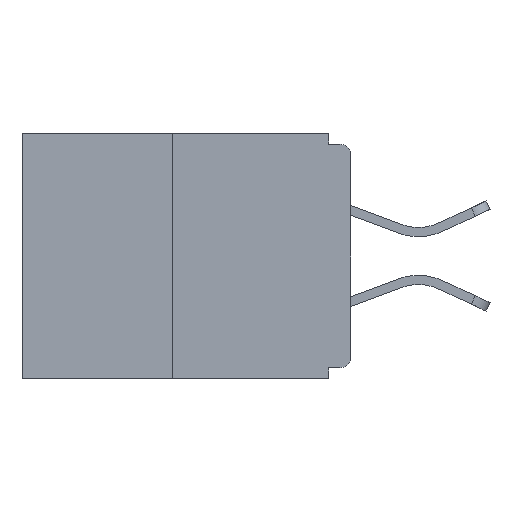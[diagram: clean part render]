
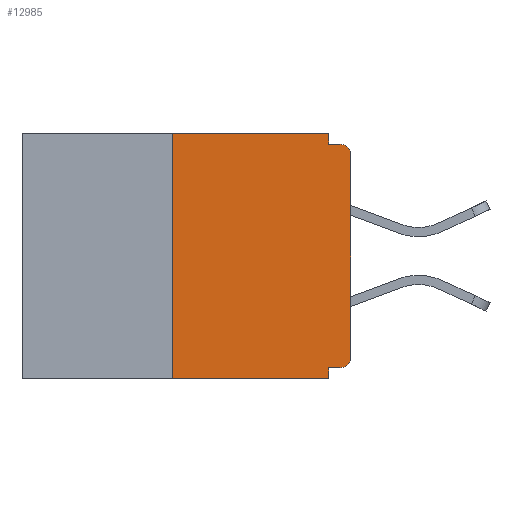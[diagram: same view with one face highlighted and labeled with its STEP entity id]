
A CAD part, left-side view. The second image highlights one B-rep face of the part: STEP entity #12985.
In plain terms, the highlighted planar face has unit normal (-1, 0, 0).
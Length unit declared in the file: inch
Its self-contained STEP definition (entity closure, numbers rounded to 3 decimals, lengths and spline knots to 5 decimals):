
#186 = CARTESIAN_POINT ( 'NONE',  ( 0., 0.25, 0. ) ) ;
#238 = VERTEX_POINT ( 'NONE', #11350 ) ;
#452 = LINE ( 'NONE', #4625, #4002 ) ;
#534 = CARTESIAN_POINT ( 'NONE',  ( 0., 0., -0.313 ) ) ;
#554 = EDGE_CURVE ( 'NONE', #14281, #17436, #20097, .T. ) ;
#616 = LINE ( 'NONE', #4988, #17726 ) ;
#737 = DIRECTION ( 'NONE',  ( 0., 0., -1. ) ) ;
#742 = EDGE_CURVE ( 'NONE', #16963, #9123, #19096, .T. ) ;
#1003 = DIRECTION ( 'NONE',  ( 0., 0., -1. ) ) ;
#1387 = DIRECTION ( 'NONE',  ( 0., 0., -1. ) ) ;
#1718 = AXIS2_PLACEMENT_3D ( 'NONE', #15982, #17653, #7843 ) ;
#1774 = DIRECTION ( 'NONE',  ( 0., 1., 0. ) ) ;
#1991 = ORIENTED_EDGE ( 'NONE', *, *, #6181, .F. ) ;
#2042 = EDGE_LOOP ( 'NONE', ( #1991, #4222, #19825, #11388, #10712, #20825, #12329, #11594, #8699, #4123 ) ) ;
#2725 = VECTOR ( 'NONE', #5269, 39.37008 ) ;
#2917 = AXIS2_PLACEMENT_3D ( 'NONE', #17072, #7532, #1003 ) ;
#3394 = LINE ( 'NONE', #186, #16691 ) ;
#3985 = CARTESIAN_POINT ( 'NONE',  ( 0., 0., -0.03 ) ) ;
#4002 = VECTOR ( 'NONE', #15808, 39.37008 ) ;
#4123 = ORIENTED_EDGE ( 'NONE', *, *, #6425, .F. ) ;
#4222 = ORIENTED_EDGE ( 'NONE', *, *, #12953, .F. ) ;
#4363 = LINE ( 'NONE', #14274, #11763 ) ;
#4625 = CARTESIAN_POINT ( 'NONE',  ( 0., 0.46, 0. ) ) ;
#4988 = CARTESIAN_POINT ( 'NONE',  ( 0., 0., -0.328 ) ) ;
#5269 = DIRECTION ( 'NONE',  ( 0., 0., -1. ) ) ;
#5302 = CARTESIAN_POINT ( 'NONE',  ( 0., 0.031, -0.343 ) ) ;
#5309 = AXIS2_PLACEMENT_3D ( 'NONE', #7139, #13700, #737 ) ;
#6152 = VERTEX_POINT ( 'NONE', #16031 ) ;
#6181 = EDGE_CURVE ( 'NONE', #11075, #6152, #452, .T. ) ;
#6289 = VECTOR ( 'NONE', #12753, 39.37008 ) ;
#6385 = VERTEX_POINT ( 'NONE', #9576 ) ;
#6425 = EDGE_CURVE ( 'NONE', #6152, #17548, #17816, .T. ) ;
#6962 = FACE_OUTER_BOUND ( 'NONE', #2042, .T. ) ;
#7139 = CARTESIAN_POINT ( 'NONE',  ( 0., 0.015, -0.03 ) ) ;
#7474 = DIRECTION ( 'NONE',  ( 0., -1., 0. ) ) ;
#7532 = DIRECTION ( 'NONE',  ( 1., 0., 0. ) ) ;
#7843 = DIRECTION ( 'NONE',  ( 0., 0., -1. ) ) ;
#8699 = ORIENTED_EDGE ( 'NONE', *, *, #20823, .F. ) ;
#9048 = EDGE_CURVE ( 'NONE', #6385, #15480, #18983, .T. ) ;
#9123 = VERTEX_POINT ( 'NONE', #5302 ) ;
#9576 = CARTESIAN_POINT ( 'NONE',  ( 0., 0.015, -0.328 ) ) ;
#10599 = LINE ( 'NONE', #11005, #6289 ) ;
#10712 = ORIENTED_EDGE ( 'NONE', *, *, #12665, .F. ) ;
#11005 = CARTESIAN_POINT ( 'NONE',  ( 0., 0., -0.015 ) ) ;
#11075 = VERTEX_POINT ( 'NONE', #20914 ) ;
#11350 = CARTESIAN_POINT ( 'NONE',  ( 0., 0.031, -0.328 ) ) ;
#11388 = ORIENTED_EDGE ( 'NONE', *, *, #18551, .F. ) ;
#11415 = CARTESIAN_POINT ( 'NONE',  ( 0., 0.015, -0.015 ) ) ;
#11487 = CARTESIAN_POINT ( 'NONE',  ( 0., 0., 0. ) ) ;
#11594 = ORIENTED_EDGE ( 'NONE', *, *, #554, .T. ) ;
#11763 = VECTOR ( 'NONE', #1387, 39.37008 ) ;
#11819 = VECTOR ( 'NONE', #16364, 39.37008 ) ;
#12077 = LINE ( 'NONE', #11487, #11819 ) ;
#12167 = CARTESIAN_POINT ( 'NONE',  ( 0., 0.25, -0.343 ) ) ;
#12329 = ORIENTED_EDGE ( 'NONE', *, *, #17417, .T. ) ;
#12665 = EDGE_CURVE ( 'NONE', #6385, #238, #616, .T. ) ;
#12753 = DIRECTION ( 'NONE',  ( 0., -1., 0. ) ) ;
#12953 = EDGE_CURVE ( 'NONE', #16963, #11075, #3394, .T. ) ;
#12985 = ADVANCED_FACE ( 'NONE', ( #6962 ), #20456, .F. ) ;
#13700 = DIRECTION ( 'NONE',  ( -1., 0., 0. ) ) ;
#13773 = DIRECTION ( 'NONE',  ( 0., 0., 1. ) ) ;
#14274 = CARTESIAN_POINT ( 'NONE',  ( 0., 0.031, -0.343 ) ) ;
#14281 = VERTEX_POINT ( 'NONE', #3985 ) ;
#14475 = VECTOR ( 'NONE', #7474, 39.37008 ) ;
#15480 = VERTEX_POINT ( 'NONE', #534 ) ;
#15808 = DIRECTION ( 'NONE',  ( 0., -1., 0. ) ) ;
#15982 = CARTESIAN_POINT ( 'NONE',  ( 0., 0.015, -0.313 ) ) ;
#16031 = CARTESIAN_POINT ( 'NONE',  ( 0., 0.031, 0. ) ) ;
#16364 = DIRECTION ( 'NONE',  ( 0., 0., 1. ) ) ;
#16677 = CARTESIAN_POINT ( 'NONE',  ( 0., 0.031, 0. ) ) ;
#16691 = VECTOR ( 'NONE', #13773, 39.37008 ) ;
#16963 = VERTEX_POINT ( 'NONE', #12167 ) ;
#17072 = CARTESIAN_POINT ( 'NONE',  ( 0., 0.46, 0. ) ) ;
#17276 = CARTESIAN_POINT ( 'NONE',  ( 0., 0.46, -0.343 ) ) ;
#17417 = EDGE_CURVE ( 'NONE', #15480, #14281, #12077, .T. ) ;
#17436 = VERTEX_POINT ( 'NONE', #11415 ) ;
#17487 = CARTESIAN_POINT ( 'NONE',  ( 0., 0.031, -0.015 ) ) ;
#17548 = VERTEX_POINT ( 'NONE', #17487 ) ;
#17653 = DIRECTION ( 'NONE',  ( -1., 0., 0. ) ) ;
#17726 = VECTOR ( 'NONE', #1774, 39.37008 ) ;
#17816 = LINE ( 'NONE', #16677, #2725 ) ;
#18551 = EDGE_CURVE ( 'NONE', #238, #9123, #4363, .T. ) ;
#18983 = CIRCLE ( 'NONE', #1718, 0.015 ) ;
#19096 = LINE ( 'NONE', #17276, #14475 ) ;
#19825 = ORIENTED_EDGE ( 'NONE', *, *, #742, .T. ) ;
#20097 = CIRCLE ( 'NONE', #5309, 0.015 ) ;
#20456 = PLANE ( 'NONE',  #2917 ) ;
#20823 = EDGE_CURVE ( 'NONE', #17548, #17436, #10599, .T. ) ;
#20825 = ORIENTED_EDGE ( 'NONE', *, *, #9048, .T. ) ;
#20914 = CARTESIAN_POINT ( 'NONE',  ( 0., 0.25, 0. ) ) ;
